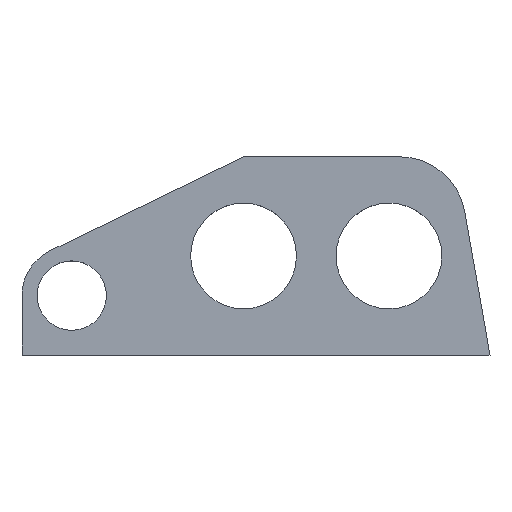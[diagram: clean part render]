
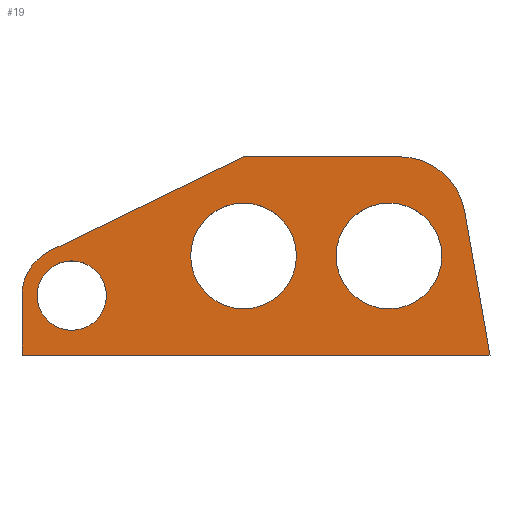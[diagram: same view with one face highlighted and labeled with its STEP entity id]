
A CAD part, top view. The second image highlights one B-rep face of the part: STEP entity #19.
In plain terms, the highlighted planar face has unit normal (0, 0, 1).
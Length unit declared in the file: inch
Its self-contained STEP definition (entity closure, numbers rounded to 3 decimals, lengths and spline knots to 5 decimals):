
#19 = ADVANCED_FACE ( 'NONE', ( #475, #553, #88, #585 ), #598, .F. ) ;
#28 = DIRECTION ( 'NONE',  ( -1., 0., 0. ) ) ;
#29 = CARTESIAN_POINT ( 'NONE',  ( 2.92236, 1.35286, -0.25 ) ) ;
#36 = ORIENTED_EDGE ( 'NONE', *, *, #433, .F. ) ;
#37 = DIRECTION ( 'NONE',  ( 0., 0., -1. ) ) ;
#43 = CIRCLE ( 'NONE', #77, 0.13125 ) ;
#44 = ORIENTED_EDGE ( 'NONE', *, *, #662, .F. ) ;
#48 = CARTESIAN_POINT ( 'NONE',  ( 2.92236, 1.35286, -0.25 ) ) ;
#58 = DIRECTION ( 'NONE',  ( 0., 0., -1. ) ) ;
#62 = VECTOR ( 'NONE', #318, 39.37008 ) ;
#66 = EDGE_CURVE ( 'NONE', #192, #96, #658, .T. ) ;
#72 = EDGE_LOOP ( 'NONE', ( #421, #36 ) ) ;
#77 = AXIS2_PLACEMENT_3D ( 'NONE', #173, #169, #557 ) ;
#85 = DIRECTION ( 'NONE',  ( 0., 0., 1. ) ) ;
#86 = AXIS2_PLACEMENT_3D ( 'NONE', #92, #697, #420 ) ;
#87 = LINE ( 'NONE', #581, #458 ) ;
#88 = FACE_BOUND ( 'NONE', #72, .T. ) ;
#89 = EDGE_CURVE ( 'NONE', #462, #95, #353, .T. ) ;
#92 = CARTESIAN_POINT ( 'NONE',  ( 4.35062, 1.85286, -0.25 ) ) ;
#93 = VECTOR ( 'NONE', #334, 39.37008 ) ;
#95 = VERTEX_POINT ( 'NONE', #606 ) ;
#96 = VERTEX_POINT ( 'NONE', #111 ) ;
#103 = CIRCLE ( 'NONE', #303, 0.2 ) ;
#105 = CARTESIAN_POINT ( 'NONE',  ( 3.11036, 1.57786, -0.25 ) ) ;
#107 = CARTESIAN_POINT ( 'NONE',  ( 4.31036, 1.72786, -0.25 ) ) ;
#108 = DIRECTION ( 'NONE',  ( 0., -1., 0. ) ) ;
#111 = CARTESIAN_POINT ( 'NONE',  ( 4.51036, 1.72786, -0.25 ) ) ;
#138 = ORIENTED_EDGE ( 'NONE', *, *, #559, .F. ) ;
#146 = ORIENTED_EDGE ( 'NONE', *, *, #66, .F. ) ;
#167 = VERTEX_POINT ( 'NONE', #668 ) ;
#168 = EDGE_CURVE ( 'NONE', #570, #694, #43, .T. ) ;
#169 = DIRECTION ( 'NONE',  ( 0., 0., 1. ) ) ;
#173 = CARTESIAN_POINT ( 'NONE',  ( 3.11036, 1.57786, -0.25 ) ) ;
#192 = VERTEX_POINT ( 'NONE', #401 ) ;
#194 = AXIS2_PLACEMENT_3D ( 'NONE', #107, #326, #325 ) ;
#202 = DIRECTION ( 'NONE',  ( 0., 1., 0. ) ) ;
#203 = EDGE_CURVE ( 'NONE', #517, #219, #533, .T. ) ;
#211 = CARTESIAN_POINT ( 'NONE',  ( 3.11036, 1.57786, -0.25 ) ) ;
#219 = VERTEX_POINT ( 'NONE', #618 ) ;
#235 = CIRCLE ( 'NONE', #592, 0.2 ) ;
#239 = CARTESIAN_POINT ( 'NONE',  ( 5.59795, 1.35286, -0.25 ) ) ;
#247 = CARTESIAN_POINT ( 'NONE',  ( 4.31036, 1.72786, -0.25 ) ) ;
#253 = VERTEX_POINT ( 'NONE', #673 ) ;
#264 = AXIS2_PLACEMENT_3D ( 'NONE', #358, #37, #108 ) ;
#276 = CARTESIAN_POINT ( 'NONE',  ( 4.5604, 2.10286, -0.25 ) ) ;
#286 = EDGE_CURVE ( 'NONE', #167, #626, #235, .T. ) ;
#291 = EDGE_LOOP ( 'NONE', ( #146, #414 ) ) ;
#295 = EDGE_CURVE ( 'NONE', #517, #333, #541, .T. ) ;
#299 = DIRECTION ( 'NONE',  ( 0., -1., 0. ) ) ;
#303 = AXIS2_PLACEMENT_3D ( 'NONE', #588, #85, #471 ) ;
#308 = CARTESIAN_POINT ( 'NONE',  ( 3.11036, 1.70911, -0.25 ) ) ;
#311 = CARTESIAN_POINT ( 'NONE',  ( 4.69264, 1.35286, -0.25 ) ) ;
#315 = CARTESIAN_POINT ( 'NONE',  ( 3.02817, 1.74694, -0.25 ) ) ;
#318 = DIRECTION ( 'NONE',  ( 0.899, 0.437, 0. ) ) ;
#325 = DIRECTION ( 'NONE',  ( 0., -1., 0. ) ) ;
#326 = DIRECTION ( 'NONE',  ( 0., 0., 1. ) ) ;
#333 = VERTEX_POINT ( 'NONE', #29 ) ;
#334 = DIRECTION ( 'NONE',  ( -0.174, 0.985, 0. ) ) ;
#343 = AXIS2_PLACEMENT_3D ( 'NONE', #247, #699, #299 ) ;
#349 = DIRECTION ( 'NONE',  ( 0., -1., 0. ) ) ;
#353 = CIRCLE ( 'NONE', #382, 0.188 ) ;
#356 = ORIENTED_EDGE ( 'NONE', *, *, #409, .F. ) ;
#358 = CARTESIAN_POINT ( 'NONE',  ( 5.59795, 1.35286, -0.25 ) ) ;
#359 = DIRECTION ( 'NONE',  ( 1., 0., 0. ) ) ;
#367 = EDGE_CURVE ( 'NONE', #219, #577, #427, .T. ) ;
#370 = CARTESIAN_POINT ( 'NONE',  ( 3.11036, 1.44661, -0.25 ) ) ;
#373 = CIRCLE ( 'NONE', #343, 0.2 ) ;
#382 = AXIS2_PLACEMENT_3D ( 'NONE', #211, #58, #601 ) ;
#386 = ORIENTED_EDGE ( 'NONE', *, *, #295, .F. ) ;
#400 = ORIENTED_EDGE ( 'NONE', *, *, #367, .T. ) ;
#401 = CARTESIAN_POINT ( 'NONE',  ( 4.11036, 1.72786, -0.25 ) ) ;
#402 = EDGE_CURVE ( 'NONE', #96, #192, #373, .T. ) ;
#406 = ORIENTED_EDGE ( 'NONE', *, *, #637, .F. ) ;
#409 = EDGE_CURVE ( 'NONE', #253, #577, #87, .T. ) ;
#412 = LINE ( 'NONE', #48, #472 ) ;
#414 = ORIENTED_EDGE ( 'NONE', *, *, #402, .F. ) ;
#418 = CARTESIAN_POINT ( 'NONE',  ( 2.92236, 1.57786, -0.25 ) ) ;
#420 = DIRECTION ( 'NONE',  ( 0., -1., 0. ) ) ;
#421 = ORIENTED_EDGE ( 'NONE', *, *, #286, .F. ) ;
#427 = CIRCLE ( 'NONE', #86, 0.25 ) ;
#433 = EDGE_CURVE ( 'NONE', #626, #167, #103, .T. ) ;
#458 = VECTOR ( 'NONE', #359, 39.37008 ) ;
#462 = VERTEX_POINT ( 'NONE', #418 ) ;
#463 = AXIS2_PLACEMENT_3D ( 'NONE', #105, #651, #590 ) ;
#465 = LINE ( 'NONE', #315, #62 ) ;
#471 = DIRECTION ( 'NONE',  ( 0., -1., 0. ) ) ;
#472 = VECTOR ( 'NONE', #202, 39.37008 ) ;
#475 = FACE_BOUND ( 'NONE', #536, .T. ) ;
#481 = CARTESIAN_POINT ( 'NONE',  ( 4.35062, 2.10286, -0.25 ) ) ;
#510 = ORIENTED_EDGE ( 'NONE', *, *, #203, .T. ) ;
#513 = CARTESIAN_POINT ( 'NONE',  ( 3.76036, 1.72786, -0.25 ) ) ;
#517 = VERTEX_POINT ( 'NONE', #311 ) ;
#533 = LINE ( 'NONE', #276, #93 ) ;
#536 = EDGE_LOOP ( 'NONE', ( #138, #613 ) ) ;
#541 = LINE ( 'NONE', #239, #603 ) ;
#553 = FACE_OUTER_BOUND ( 'NONE', #595, .T. ) ;
#557 = DIRECTION ( 'NONE',  ( 0., -1., 0. ) ) ;
#559 = EDGE_CURVE ( 'NONE', #694, #570, #649, .T. ) ;
#570 = VERTEX_POINT ( 'NONE', #308 ) ;
#571 = DIRECTION ( 'NONE',  ( 0., 0., 1. ) ) ;
#577 = VERTEX_POINT ( 'NONE', #481 ) ;
#581 = CARTESIAN_POINT ( 'NONE',  ( 4.5604, 2.10286, -0.25 ) ) ;
#585 = FACE_BOUND ( 'NONE', #291, .T. ) ;
#588 = CARTESIAN_POINT ( 'NONE',  ( 3.76036, 1.72786, -0.25 ) ) ;
#590 = DIRECTION ( 'NONE',  ( 0., -1., 0. ) ) ;
#592 = AXIS2_PLACEMENT_3D ( 'NONE', #513, #571, #349 ) ;
#595 = EDGE_LOOP ( 'NONE', ( #510, #400, #356, #406, #650, #44, #386 ) ) ;
#598 = PLANE ( 'NONE',  #264 ) ;
#601 = DIRECTION ( 'NONE',  ( 0., -1., 0. ) ) ;
#603 = VECTOR ( 'NONE', #28, 39.37008 ) ;
#606 = CARTESIAN_POINT ( 'NONE',  ( 3.02817, 1.74694, -0.25 ) ) ;
#613 = ORIENTED_EDGE ( 'NONE', *, *, #168, .F. ) ;
#618 = CARTESIAN_POINT ( 'NONE',  ( 4.59683, 1.89627, -0.25 ) ) ;
#626 = VERTEX_POINT ( 'NONE', #705 ) ;
#637 = EDGE_CURVE ( 'NONE', #95, #253, #465, .T. ) ;
#649 = CIRCLE ( 'NONE', #463, 0.13125 ) ;
#650 = ORIENTED_EDGE ( 'NONE', *, *, #89, .F. ) ;
#651 = DIRECTION ( 'NONE',  ( 0., 0., 1. ) ) ;
#658 = CIRCLE ( 'NONE', #194, 0.2 ) ;
#662 = EDGE_CURVE ( 'NONE', #333, #462, #412, .T. ) ;
#668 = CARTESIAN_POINT ( 'NONE',  ( 3.56036, 1.72786, -0.25 ) ) ;
#673 = CARTESIAN_POINT ( 'NONE',  ( 3.76036, 2.10286, -0.25 ) ) ;
#694 = VERTEX_POINT ( 'NONE', #370 ) ;
#697 = DIRECTION ( 'NONE',  ( 0., 0., 1. ) ) ;
#699 = DIRECTION ( 'NONE',  ( 0., 0., 1. ) ) ;
#705 = CARTESIAN_POINT ( 'NONE',  ( 3.96036, 1.72786, -0.25 ) ) ;
